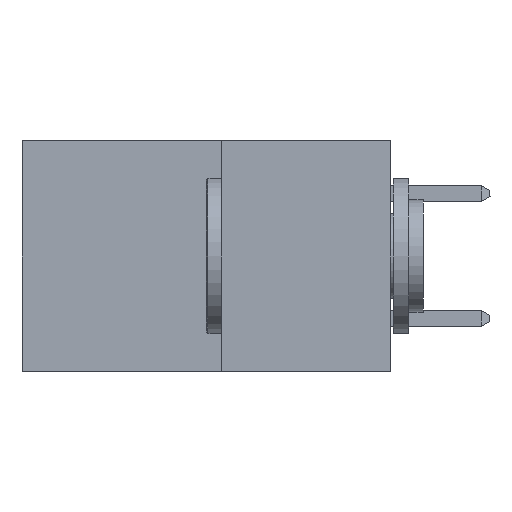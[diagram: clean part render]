
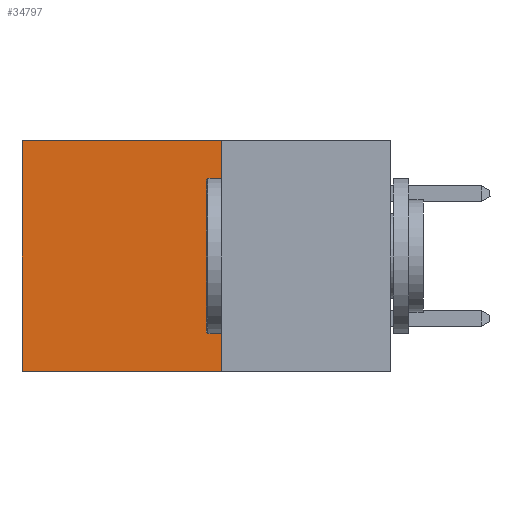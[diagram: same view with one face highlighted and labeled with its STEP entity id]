
A CAD part, left-side view. The second image highlights one B-rep face of the part: STEP entity #34797.
In plain terms, the highlighted planar face has unit normal (-1, 0, 0).
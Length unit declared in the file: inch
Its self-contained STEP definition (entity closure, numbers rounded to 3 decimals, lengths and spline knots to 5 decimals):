
#191 = FACE_OUTER_BOUND ( 'NONE', #4219, .T. ) ;
#1737 = EDGE_CURVE ( 'NONE', #32782, #22352, #15535, .T. ) ;
#2908 = EDGE_CURVE ( 'NONE', #31603, #21173, #18372, .T. ) ;
#3332 = EDGE_CURVE ( 'NONE', #31603, #32782, #11896, .T. ) ;
#4219 = EDGE_LOOP ( 'NONE', ( #6954, #21209, #26754, #22297 ) ) ;
#4525 = DIRECTION ( 'NONE',  ( 0., 0., -1. ) ) ;
#4544 = LINE ( 'NONE', #12861, #24614 ) ;
#6954 = ORIENTED_EDGE ( 'NONE', *, *, #24483, .T. ) ;
#7345 = VECTOR ( 'NONE', #9969, 39.37008 ) ;
#7536 = DIRECTION ( 'NONE',  ( 0., 1., 0. ) ) ;
#8539 = AXIS2_PLACEMENT_3D ( 'NONE', #16893, #14276, #33155 ) ;
#9259 = DIRECTION ( 'NONE',  ( 0., 0., -1. ) ) ;
#9749 = CARTESIAN_POINT ( 'NONE',  ( 0.277, 0.27, 0. ) ) ;
#9969 = DIRECTION ( 'NONE',  ( 0., 1., 0. ) ) ;
#10063 = CARTESIAN_POINT ( 'NONE',  ( 0.277, 0.27, -0.37 ) ) ;
#10369 = CARTESIAN_POINT ( 'NONE',  ( 0.277, 0.27, -0.37 ) ) ;
#11056 = VECTOR ( 'NONE', #7536, 39.37008 ) ;
#11498 = PLANE ( 'NONE',  #8539 ) ;
#11896 = LINE ( 'NONE', #10369, #19193 ) ;
#12861 = CARTESIAN_POINT ( 'NONE',  ( 0.277, 0.59, -0.37 ) ) ;
#14276 = DIRECTION ( 'NONE',  ( 1., 0., 0. ) ) ;
#15535 = LINE ( 'NONE', #10063, #7345 ) ;
#16893 = CARTESIAN_POINT ( 'NONE',  ( 0.277, 0.27, -0.37 ) ) ;
#18372 = LINE ( 'NONE', #9749, #11056 ) ;
#19193 = VECTOR ( 'NONE', #9259, 39.37008 ) ;
#20030 = CARTESIAN_POINT ( 'NONE',  ( 0.277, 0.59, 0. ) ) ;
#21173 = VERTEX_POINT ( 'NONE', #20030 ) ;
#21209 = ORIENTED_EDGE ( 'NONE', *, *, #1737, .F. ) ;
#22297 = ORIENTED_EDGE ( 'NONE', *, *, #2908, .T. ) ;
#22352 = VERTEX_POINT ( 'NONE', #25007 ) ;
#24483 = EDGE_CURVE ( 'NONE', #21173, #22352, #4544, .T. ) ;
#24614 = VECTOR ( 'NONE', #4525, 39.37008 ) ;
#25007 = CARTESIAN_POINT ( 'NONE',  ( 0.277, 0.59, -0.37 ) ) ;
#26754 = ORIENTED_EDGE ( 'NONE', *, *, #3332, .F. ) ;
#31603 = VERTEX_POINT ( 'NONE', #35182 ) ;
#32782 = VERTEX_POINT ( 'NONE', #33740 ) ;
#33155 = DIRECTION ( 'NONE',  ( 0., 0., -1. ) ) ;
#33740 = CARTESIAN_POINT ( 'NONE',  ( 0.277, 0.27, -0.37 ) ) ;
#34797 = ADVANCED_FACE ( 'NONE', ( #191 ), #11498, .F. ) ;
#35182 = CARTESIAN_POINT ( 'NONE',  ( 0.277, 0.27, 0. ) ) ;
